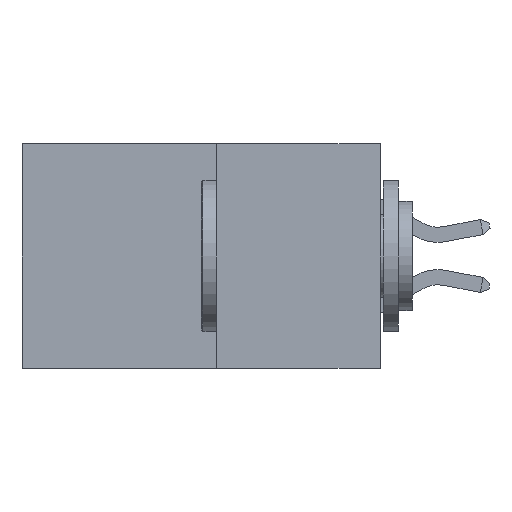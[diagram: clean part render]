
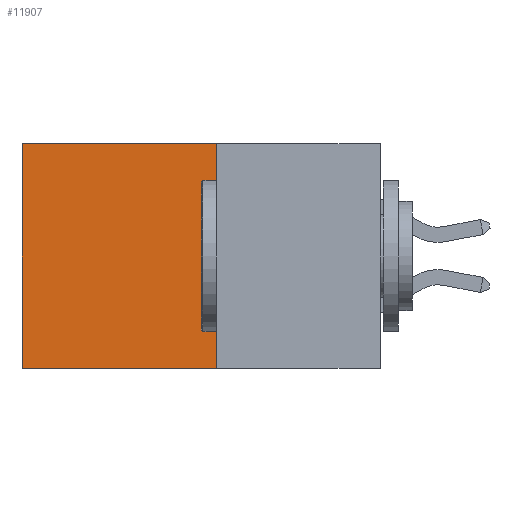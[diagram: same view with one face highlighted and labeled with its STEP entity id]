
A CAD part, left-side view. The second image highlights one B-rep face of the part: STEP entity #11907.
In plain terms, the highlighted planar face has unit normal (-1, 0, 0).
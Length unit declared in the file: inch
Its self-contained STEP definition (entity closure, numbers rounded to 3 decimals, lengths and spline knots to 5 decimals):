
#77 = CARTESIAN_POINT ( 'NONE',  ( 0.277, 0.59, -0.37 ) ) ;
#791 = DIRECTION ( 'NONE',  ( 0., 0., -1. ) ) ;
#940 = VECTOR ( 'NONE', #12615, 39.37008 ) ;
#2389 = EDGE_CURVE ( 'NONE', #22077, #10950, #5933, .T. ) ;
#3629 = CARTESIAN_POINT ( 'NONE',  ( 0.277, 0.59, 0. ) ) ;
#3735 = VECTOR ( 'NONE', #11212, 39.37008 ) ;
#3745 = CARTESIAN_POINT ( 'NONE',  ( 0.277, 0.27, -0.37 ) ) ;
#4783 = LINE ( 'NONE', #10605, #22983 ) ;
#5083 = EDGE_CURVE ( 'NONE', #7999, #5516, #8744, .T. ) ;
#5516 = VERTEX_POINT ( 'NONE', #3629 ) ;
#5933 = LINE ( 'NONE', #3745, #940 ) ;
#6741 = CARTESIAN_POINT ( 'NONE',  ( 0.277, 0.27, -0.37 ) ) ;
#7626 = CARTESIAN_POINT ( 'NONE',  ( 0.277, 0.27, 0. ) ) ;
#7999 = VERTEX_POINT ( 'NONE', #7626 ) ;
#8592 = ORIENTED_EDGE ( 'NONE', *, *, #21905, .F. ) ;
#8744 = LINE ( 'NONE', #11323, #3735 ) ;
#10605 = CARTESIAN_POINT ( 'NONE',  ( 0.277, 0.27, -0.37 ) ) ;
#10950 = VERTEX_POINT ( 'NONE', #77 ) ;
#11212 = DIRECTION ( 'NONE',  ( 0., 1., 0. ) ) ;
#11323 = CARTESIAN_POINT ( 'NONE',  ( 0.277, 0.27, 0. ) ) ;
#11907 = ADVANCED_FACE ( 'NONE', ( #16775 ), #20941, .F. ) ;
#12002 = DIRECTION ( 'NONE',  ( 1., 0., 0. ) ) ;
#12097 = LINE ( 'NONE', #17380, #16784 ) ;
#12421 = DIRECTION ( 'NONE',  ( 0., 0., -1. ) ) ;
#12615 = DIRECTION ( 'NONE',  ( 0., 1., 0. ) ) ;
#12921 = ORIENTED_EDGE ( 'NONE', *, *, #2389, .F. ) ;
#14548 = EDGE_LOOP ( 'NONE', ( #17040, #12921, #8592, #18211 ) ) ;
#16775 = FACE_OUTER_BOUND ( 'NONE', #14548, .T. ) ;
#16784 = VECTOR ( 'NONE', #19225, 39.37008 ) ;
#17040 = ORIENTED_EDGE ( 'NONE', *, *, #21769, .T. ) ;
#17263 = CARTESIAN_POINT ( 'NONE',  ( 0.277, 0.27, -0.37 ) ) ;
#17380 = CARTESIAN_POINT ( 'NONE',  ( 0.277, 0.59, -0.37 ) ) ;
#18211 = ORIENTED_EDGE ( 'NONE', *, *, #5083, .T. ) ;
#19225 = DIRECTION ( 'NONE',  ( 0., 0., -1. ) ) ;
#19384 = AXIS2_PLACEMENT_3D ( 'NONE', #17263, #12002, #791 ) ;
#20941 = PLANE ( 'NONE',  #19384 ) ;
#21769 = EDGE_CURVE ( 'NONE', #5516, #10950, #12097, .T. ) ;
#21905 = EDGE_CURVE ( 'NONE', #7999, #22077, #4783, .T. ) ;
#22077 = VERTEX_POINT ( 'NONE', #6741 ) ;
#22983 = VECTOR ( 'NONE', #12421, 39.37008 ) ;
